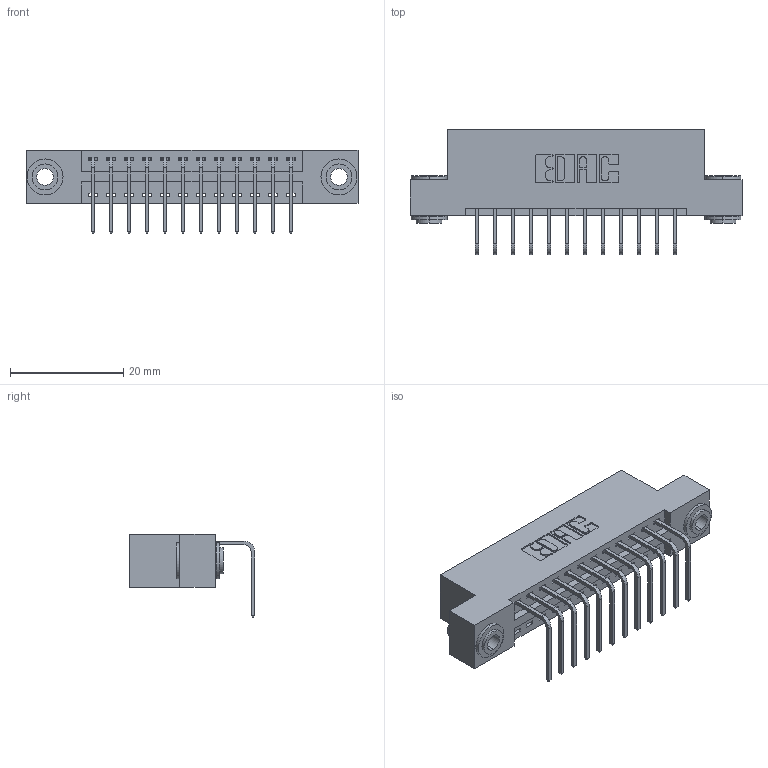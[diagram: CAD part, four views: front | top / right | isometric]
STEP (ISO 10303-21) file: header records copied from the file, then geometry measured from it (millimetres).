
FILE_DESCRIPTION (( 'STEP AP203' ), '1' );
FILE_NAME ('346-012-558-103.STEP', '2022-05-05T03:21:36', ( '' ), ( '' ), 'SwSTEP 2.0', 'SolidWorks 2020', '' );
FILE_SCHEMA (( 'CONFIG_CONTROL_DESIGN' ));
Length unit declared in the file: inch
Products named in the file (4): 345-250-002_345-250-002-102; 346 Part_Flush Mounting Lugs - 0.156 Dia-TH; 346-012-558-103; 345-292-001_558 Tail - 2
Assembly tree (15 placements, depth 2):
  346-012-558-103
    346 Part_Flush Mounting Lugs - 0.156 Dia-TH
    345-292-001_558 Tail - 2  x12
    345-250-002_345-250-002-102  x2
Bounding box: 58.67 x 22.16 x 14.73 mm (x, y, z)
Volume: 5451 mm3; surface area: 6979.3 mm2
Topology: 15 solids, 15 shells, 894 faces, 2625 edges, 1730 vertices
Faces by surface type: plane 604, cylinder 282, cone 8
Entity records: 12636 total; most frequent: CARTESIAN_POINT 2157, ORIENTED_EDGE 2094, DIRECTION 1969, EDGE_CURVE 1047, VECTOR 843, LINE 843, VERTEX_POINT 694, AXIS2_PLACEMENT_3D 563
